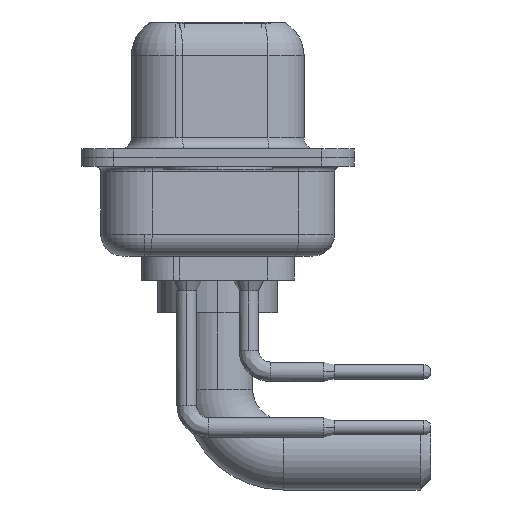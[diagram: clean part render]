
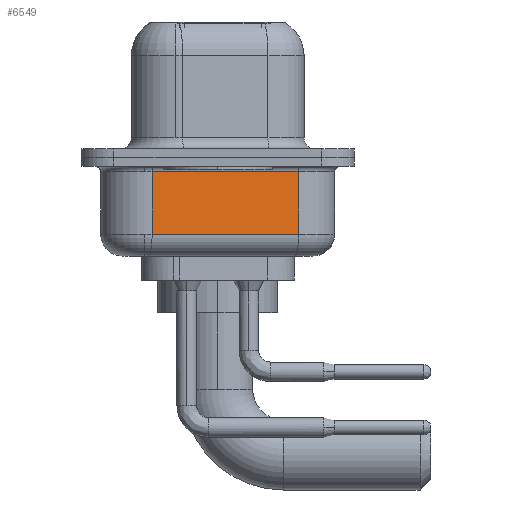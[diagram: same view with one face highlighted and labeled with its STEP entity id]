
A CAD part, left-side view. The second image highlights one B-rep face of the part: STEP entity #6549.
In plain terms, the highlighted planar face has unit normal (-0.985, -0.174, 0).
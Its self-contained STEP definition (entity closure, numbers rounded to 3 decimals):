
#437 = ORIENTED_EDGE ( 'NONE', *, *, #3433, .T. ) ;
#1101 = CARTESIAN_POINT ( 'NONE',  ( 2.88, 3.003, -4.5 ) ) ;
#1127 = VECTOR ( 'NONE', #13269, 1000. ) ;
#1677 = LINE ( 'NONE', #11906, #1127 ) ;
#1810 = VERTEX_POINT ( 'NONE', #4436 ) ;
#2160 = CARTESIAN_POINT ( 'NONE',  ( 4.062, -3.697, -4.5 ) ) ;
#2505 = CARTESIAN_POINT ( 'NONE',  ( 2.88, 3.003, -3.5 ) ) ;
#2643 = CARTESIAN_POINT ( 'NONE',  ( 2.88, 3.003, -4.5 ) ) ;
#2881 = LINE ( 'NONE', #4299, #12194 ) ;
#3027 = VECTOR ( 'NONE', #10885, 1000. ) ;
#3433 = EDGE_CURVE ( 'NONE', #9037, #1810, #9696, .T. ) ;
#3817 = AXIS2_PLACEMENT_3D ( 'NONE', #2643, #7746, #12886 ) ;
#3870 = LINE ( 'NONE', #1101, #9360 ) ;
#4197 = CARTESIAN_POINT ( 'NONE',  ( 4.062, -3.697, -3.5 ) ) ;
#4299 = CARTESIAN_POINT ( 'NONE',  ( 2.88, 3.003, -0.65 ) ) ;
#4436 = CARTESIAN_POINT ( 'NONE',  ( 4.062, -3.697, -0.65 ) ) ;
#4613 = ORIENTED_EDGE ( 'NONE', *, *, #16538, .T. ) ;
#4615 = VERTEX_POINT ( 'NONE', #14938 ) ;
#6531 = ORIENTED_EDGE ( 'NONE', *, *, #8723, .T. ) ;
#6549 = ADVANCED_FACE ( 'NONE', ( #9012 ), #14162, .F. ) ;
#7746 = DIRECTION ( 'NONE',  ( 0.985, 0.174, 0. ) ) ;
#8723 = EDGE_CURVE ( 'NONE', #1810, #4615, #2881, .T. ) ;
#8980 = DIRECTION ( 'NONE',  ( 0., 0., 1. ) ) ;
#9012 = FACE_OUTER_BOUND ( 'NONE', #15573, .T. ) ;
#9037 = VERTEX_POINT ( 'NONE', #4197 ) ;
#9360 = VECTOR ( 'NONE', #8980, 1000. ) ;
#9432 = VERTEX_POINT ( 'NONE', #2505 ) ;
#9696 = LINE ( 'NONE', #2160, #3027 ) ;
#10594 = DIRECTION ( 'NONE',  ( -0.174, 0.985, 0. ) ) ;
#10885 = DIRECTION ( 'NONE',  ( 0., 0., 1. ) ) ;
#11906 = CARTESIAN_POINT ( 'NONE',  ( 2.88, 3.003, -3.5 ) ) ;
#12194 = VECTOR ( 'NONE', #10594, 1000. ) ;
#12886 = DIRECTION ( 'NONE',  ( -0.174, 0.985, 0. ) ) ;
#13269 = DIRECTION ( 'NONE',  ( 0.174, -0.985, 0. ) ) ;
#14081 = EDGE_CURVE ( 'NONE', #9432, #4615, #3870, .T. ) ;
#14162 = PLANE ( 'NONE',  #3817 ) ;
#14676 = ORIENTED_EDGE ( 'NONE', *, *, #14081, .F. ) ;
#14938 = CARTESIAN_POINT ( 'NONE',  ( 2.88, 3.003, -0.65 ) ) ;
#15573 = EDGE_LOOP ( 'NONE', ( #14676, #4613, #437, #6531 ) ) ;
#16538 = EDGE_CURVE ( 'NONE', #9432, #9037, #1677, .T. ) ;
